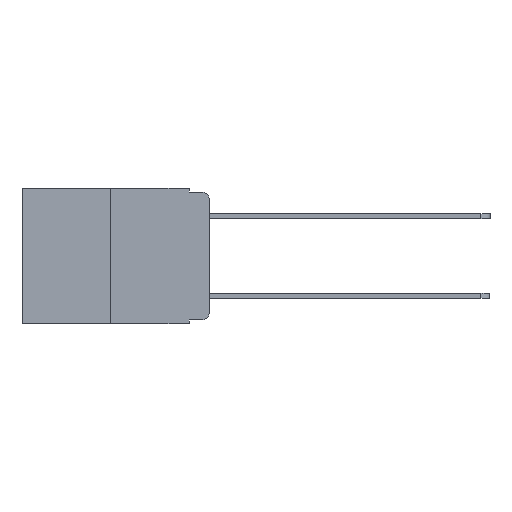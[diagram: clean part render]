
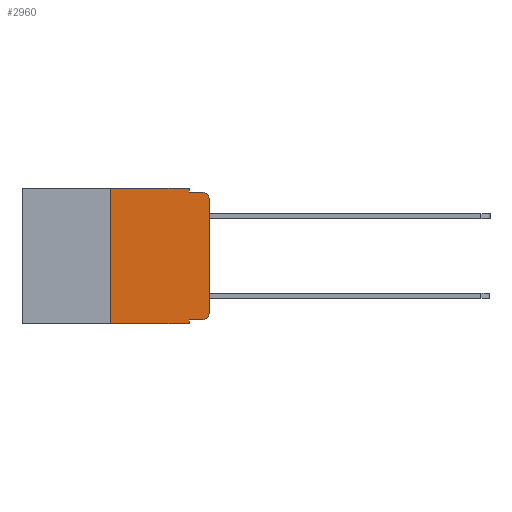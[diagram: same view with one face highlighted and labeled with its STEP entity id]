
A CAD part, left-side view. The second image highlights one B-rep face of the part: STEP entity #2960.
In plain terms, the highlighted planar face has unit normal (-1, 0, 0).
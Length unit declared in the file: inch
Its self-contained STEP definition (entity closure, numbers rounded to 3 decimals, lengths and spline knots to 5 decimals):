
#238 = ORIENTED_EDGE ( 'NONE', *, *, #1849, .F. ) ;
#249 = ORIENTED_EDGE ( 'NONE', *, *, #9161, .T. ) ;
#257 = LINE ( 'NONE', #7770, #7391 ) ;
#383 = ORIENTED_EDGE ( 'NONE', *, *, #1810, .F. ) ;
#515 = VERTEX_POINT ( 'NONE', #9378 ) ;
#666 = ORIENTED_EDGE ( 'NONE', *, *, #10434, .T. ) ;
#750 = ORIENTED_EDGE ( 'NONE', *, *, #1929, .F. ) ;
#830 = VECTOR ( 'NONE', #10952, 39.37008 ) ;
#956 = VERTEX_POINT ( 'NONE', #5503 ) ;
#1197 = ORIENTED_EDGE ( 'NONE', *, *, #6285, .F. ) ;
#1518 = ORIENTED_EDGE ( 'NONE', *, *, #2171, .T. ) ;
#1531 = LINE ( 'NONE', #3496, #10098 ) ;
#1787 = EDGE_CURVE ( 'NONE', #7136, #956, #1839, .T. ) ;
#1810 = EDGE_CURVE ( 'NONE', #9604, #956, #1531, .T. ) ;
#1830 = ORIENTED_EDGE ( 'NONE', *, *, #2418, .T. ) ;
#1839 = CIRCLE ( 'NONE', #5971, 0.02 ) ;
#1849 = EDGE_CURVE ( 'NONE', #515, #9604, #7863, .T. ) ;
#1929 = EDGE_CURVE ( 'NONE', #9107, #9903, #257, .T. ) ;
#2120 = LINE ( 'NONE', #3938, #8791 ) ;
#2151 = EDGE_CURVE ( 'NONE', #8774, #6964, #2120, .T. ) ;
#2171 = EDGE_CURVE ( 'NONE', #8774, #6611, #4568, .T. ) ;
#2279 = CARTESIAN_POINT ( 'NONE',  ( 0., 0., -0.313 ) ) ;
#2418 = EDGE_CURVE ( 'NONE', #6611, #7782, #10265, .T. ) ;
#2513 = DIRECTION ( 'NONE',  ( 0., 0., -1. ) ) ;
#2652 = DIRECTION ( 'NONE',  ( 0., -1., 0. ) ) ;
#2783 = DIRECTION ( 'NONE',  ( 0., 0., -1. ) ) ;
#2797 = CARTESIAN_POINT ( 'NONE',  ( 0., 0.051, 0. ) ) ;
#2883 = CARTESIAN_POINT ( 'NONE',  ( 0., 0.473, 0. ) ) ;
#2960 = ADVANCED_FACE ( 'NONE', ( #4872 ), #8128, .F. ) ;
#3365 = CARTESIAN_POINT ( 'NONE',  ( 0., 0.02, -0.313 ) ) ;
#3460 = VECTOR ( 'NONE', #2783, 39.37008 ) ;
#3496 = CARTESIAN_POINT ( 'NONE',  ( 0., 0.051, -0.01 ) ) ;
#3524 = DIRECTION ( 'NONE',  ( 0., -1., 0. ) ) ;
#3539 = DIRECTION ( 'NONE',  ( 0., 0., -1. ) ) ;
#3541 = DIRECTION ( 'NONE',  ( -1., 0., 0. ) ) ;
#3568 = CARTESIAN_POINT ( 'NONE',  ( 0., 0.02, -0.03 ) ) ;
#3938 = CARTESIAN_POINT ( 'NONE',  ( 0., 0.051, 0. ) ) ;
#4287 = VECTOR ( 'NONE', #2652, 39.37008 ) ;
#4568 = LINE ( 'NONE', #5709, #4287 ) ;
#4872 = FACE_OUTER_BOUND ( 'NONE', #7785, .T. ) ;
#4937 = LINE ( 'NONE', #2883, #10662 ) ;
#5156 = AXIS2_PLACEMENT_3D ( 'NONE', #9100, #7588, #9415 ) ;
#5459 = CARTESIAN_POINT ( 'NONE',  ( 0., 0.25, -0.343 ) ) ;
#5463 = AXIS2_PLACEMENT_3D ( 'NONE', #3365, #10408, #10357 ) ;
#5503 = CARTESIAN_POINT ( 'NONE',  ( 0., 0.02, -0.01 ) ) ;
#5524 = LINE ( 'NONE', #10446, #9640 ) ;
#5709 = CARTESIAN_POINT ( 'NONE',  ( 0., 0.051, -0.333 ) ) ;
#5852 = CARTESIAN_POINT ( 'NONE',  ( 0., 0.25, 0. ) ) ;
#5873 = DIRECTION ( 'NONE',  ( 0., 0., 1. ) ) ;
#5971 = AXIS2_PLACEMENT_3D ( 'NONE', #3568, #3541, #3539 ) ;
#6285 = EDGE_CURVE ( 'NONE', #9903, #515, #4937, .T. ) ;
#6559 = CARTESIAN_POINT ( 'NONE',  ( 0., 0.02, -0.333 ) ) ;
#6611 = VERTEX_POINT ( 'NONE', #6559 ) ;
#6964 = VERTEX_POINT ( 'NONE', #10699 ) ;
#7136 = VERTEX_POINT ( 'NONE', #10170 ) ;
#7147 = DIRECTION ( 'NONE',  ( 0., -1., 0. ) ) ;
#7342 = DIRECTION ( 'NONE',  ( 0., 0., 1. ) ) ;
#7391 = VECTOR ( 'NONE', #7342, 39.37008 ) ;
#7588 = DIRECTION ( 'NONE',  ( 1., 0., 0. ) ) ;
#7770 = CARTESIAN_POINT ( 'NONE',  ( 0., 0.25, 0. ) ) ;
#7782 = VERTEX_POINT ( 'NONE', #2279 ) ;
#7785 = EDGE_LOOP ( 'NONE', ( #666, #9669, #383, #238, #1197, #750, #249, #7854, #1518, #1830 ) ) ;
#7854 = ORIENTED_EDGE ( 'NONE', *, *, #2151, .F. ) ;
#7863 = LINE ( 'NONE', #2797, #3460 ) ;
#8128 = PLANE ( 'NONE',  #5156 ) ;
#8774 = VERTEX_POINT ( 'NONE', #10260 ) ;
#8791 = VECTOR ( 'NONE', #2513, 39.37008 ) ;
#9100 = CARTESIAN_POINT ( 'NONE',  ( 0., 0.473, 0. ) ) ;
#9107 = VERTEX_POINT ( 'NONE', #5459 ) ;
#9161 = EDGE_CURVE ( 'NONE', #9107, #6964, #9550, .T. ) ;
#9259 = CARTESIAN_POINT ( 'NONE',  ( 0., 0.051, -0.01 ) ) ;
#9378 = CARTESIAN_POINT ( 'NONE',  ( 0., 0.051, 0. ) ) ;
#9415 = DIRECTION ( 'NONE',  ( 0., 0., -1. ) ) ;
#9550 = LINE ( 'NONE', #10186, #830 ) ;
#9604 = VERTEX_POINT ( 'NONE', #9259 ) ;
#9640 = VECTOR ( 'NONE', #5873, 39.37008 ) ;
#9669 = ORIENTED_EDGE ( 'NONE', *, *, #1787, .T. ) ;
#9903 = VERTEX_POINT ( 'NONE', #5852 ) ;
#10098 = VECTOR ( 'NONE', #3524, 39.37008 ) ;
#10170 = CARTESIAN_POINT ( 'NONE',  ( 0., 0., -0.03 ) ) ;
#10186 = CARTESIAN_POINT ( 'NONE',  ( 0., 0.473, -0.343 ) ) ;
#10260 = CARTESIAN_POINT ( 'NONE',  ( 0., 0.051, -0.333 ) ) ;
#10265 = CIRCLE ( 'NONE', #5463, 0.02 ) ;
#10357 = DIRECTION ( 'NONE',  ( 0., 0., -1. ) ) ;
#10408 = DIRECTION ( 'NONE',  ( -1., 0., 0. ) ) ;
#10434 = EDGE_CURVE ( 'NONE', #7782, #7136, #5524, .T. ) ;
#10446 = CARTESIAN_POINT ( 'NONE',  ( 0., 0., 0. ) ) ;
#10662 = VECTOR ( 'NONE', #7147, 39.37008 ) ;
#10699 = CARTESIAN_POINT ( 'NONE',  ( 0., 0.051, -0.343 ) ) ;
#10952 = DIRECTION ( 'NONE',  ( 0., -1., 0. ) ) ;
